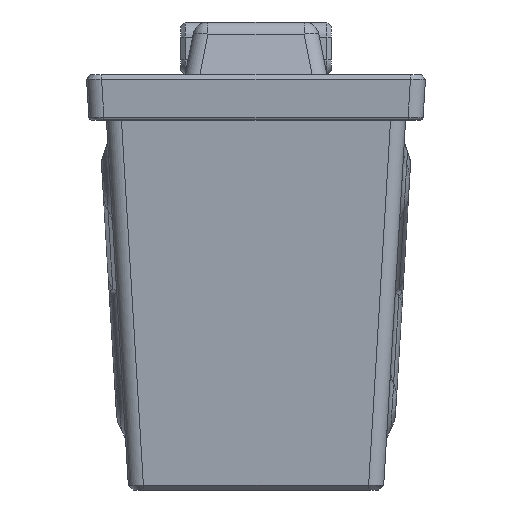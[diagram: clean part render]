
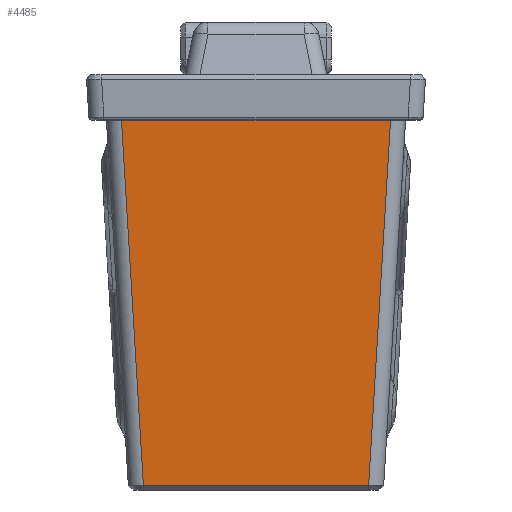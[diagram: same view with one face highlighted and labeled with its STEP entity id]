
A CAD part, front view. The second image highlights one B-rep face of the part: STEP entity #4485.
In plain terms, the highlighted planar face has unit normal (0, -0.998, -0.06).
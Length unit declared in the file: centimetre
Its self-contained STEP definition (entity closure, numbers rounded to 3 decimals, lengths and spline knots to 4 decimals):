
#97=B_SPLINE_CURVE_WITH_KNOTS($,3,(#7843,#7844,#7845,#7846),
 .UNSPECIFIED.,.F.,.F.,(4,4),(-0.7836,-0.766),
 .UNSPECIFIED.);
#98=B_SPLINE_CURVE_WITH_KNOTS($,3,(#7849,#7850,#7851,#7852),
 .UNSPECIFIED.,.F.,.F.,(4,4),(0.766,0.7836),
 .UNSPECIFIED.);
#162=PLANE($,#4884);
#254=LINE($,#6752,#598);
#271=LINE($,#6907,#615);
#309=LINE($,#7720,#653);
#324=LINE($,#7848,#668);
#598=VECTOR($,#5293,3.5931);
#615=VECTOR($,#5344,5.0948);
#653=VECTOR($,#5594,5.0948);
#668=VECTOR($,#5661,2.9767);
#1126=FACE_OUTER_BOUND($,#1419,.T.);
#1419=EDGE_LOOP($,(#3413,#3414,#3415,#3416,#3417,#3418));
#1936=VERTEX_POINT($,#6742);
#1938=VERTEX_POINT($,#6750);
#1963=VERTEX_POINT($,#6906);
#2036=VERTEX_POINT($,#7714);
#2061=VERTEX_POINT($,#7842);
#2062=VERTEX_POINT($,#7847);
#2349=EDGE_CURVE($,#1938,#1936,#254,.T.);
#2382=EDGE_CURVE($,#1936,#1963,#271,.T.);
#2510=EDGE_CURVE($,#2036,#1938,#309,.T.);
#2548=EDGE_CURVE($,#2061,#2036,#97,.T.);
#2549=EDGE_CURVE($,#2062,#2061,#324,.T.);
#2550=EDGE_CURVE($,#1963,#2062,#98,.T.);
#3413=ORIENTED_EDGE($,*,*,#2349,.F.);
#3414=ORIENTED_EDGE($,*,*,#2510,.F.);
#3415=ORIENTED_EDGE($,*,*,#2548,.F.);
#3416=ORIENTED_EDGE($,*,*,#2549,.F.);
#3417=ORIENTED_EDGE($,*,*,#2550,.F.);
#3418=ORIENTED_EDGE($,*,*,#2382,.F.);
#4485=ADVANCED_FACE($,(#1126),#162,.F.);
#4884=AXIS2_PLACEMENT_3D($,#7841,#5659,#5660);
#5293=DIRECTION($,(1.,0.,0.));
#5344=DIRECTION($,(-0.06,0.06,-0.996));
#5594=DIRECTION($,(-0.06,-0.06,0.996));
#5659=DIRECTION('center_axis',(0.,0.998,0.06));
#5660=DIRECTION('ref_axis',(0.,-0.06,0.998));
#5661=DIRECTION($,(-1.,0.,0.));
#6742=CARTESIAN_POINT('',(-3.2035,0.0038,4.9364));
#6750=CARTESIAN_POINT('',(-6.7965,0.0038,4.9364));
#6752=CARTESIAN_POINT($,(-5.,0.0038,4.9364));
#6906=CARTESIAN_POINT('',(-3.508,0.3084,-0.1401));
#6907=CARTESIAN_POINT($,(-3.4552,0.2555,0.7414));
#7714=CARTESIAN_POINT('',(-6.492,0.3084,-0.1401));
#7720=CARTESIAN_POINT($,(-6.5448,0.2555,0.7414));
#7841=CARTESIAN_POINT('Origin',(-5.,0.2401,0.9982));
#7842=CARTESIAN_POINT('',(-6.4884,0.3084,-0.1401));
#7843=CARTESIAN_POINT('Ctrl Pts',(-6.4884,0.3084,-0.1401));
#7844=CARTESIAN_POINT('Ctrl Pts',(-6.4896,0.3084,-0.1401));
#7845=CARTESIAN_POINT('Ctrl Pts',(-6.4908,0.3084,-0.1401));
#7846=CARTESIAN_POINT('Ctrl Pts',(-6.492,0.3084,-0.1401));
#7847=CARTESIAN_POINT('',(-3.5116,0.3084,-0.1401));
#7848=CARTESIAN_POINT($,(-5.,0.3084,-0.1401));
#7849=CARTESIAN_POINT('Ctrl Pts',(-3.508,0.3084,-0.1401));
#7850=CARTESIAN_POINT('Ctrl Pts',(-3.5092,0.3084,-0.1401));
#7851=CARTESIAN_POINT('Ctrl Pts',(-3.5104,0.3084,-0.1401));
#7852=CARTESIAN_POINT('Ctrl Pts',(-3.5116,0.3084,-0.1401));
